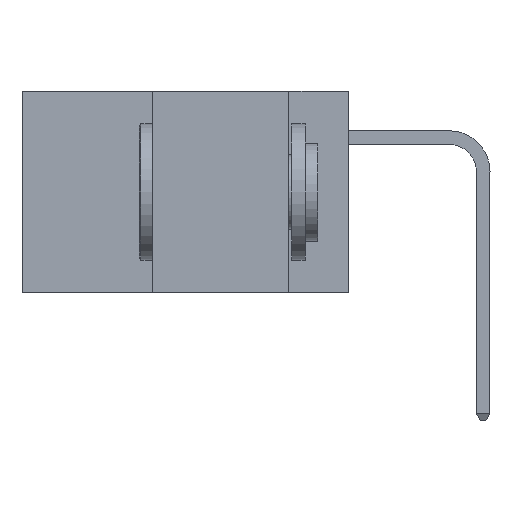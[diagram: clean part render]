
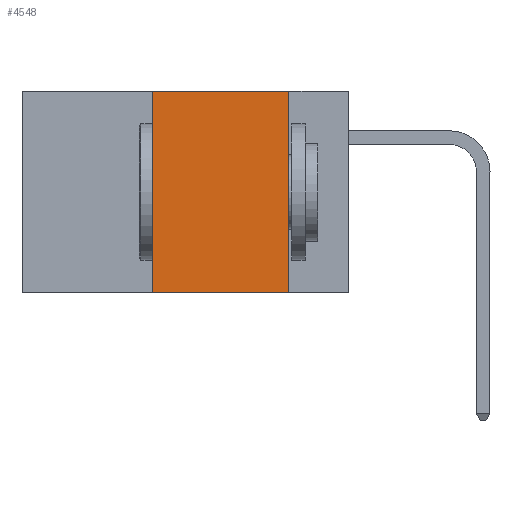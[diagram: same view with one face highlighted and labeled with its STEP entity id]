
A CAD part, left-side view. The second image highlights one B-rep face of the part: STEP entity #4548.
In plain terms, the highlighted planar face has unit normal (-1, 0, 0).
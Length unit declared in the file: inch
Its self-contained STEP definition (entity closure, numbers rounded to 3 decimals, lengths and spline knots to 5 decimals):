
#1615 = DIRECTION ( 'NONE',  ( 0., 0., -1. ) ) ;
#1675 = VECTOR ( 'NONE', #27861, 39.37008 ) ;
#3706 = LINE ( 'NONE', #6561, #33456 ) ;
#4021 = CARTESIAN_POINT ( 'NONE',  ( 0., 0.11, -0.37 ) ) ;
#4035 = CARTESIAN_POINT ( 'NONE',  ( 0., 0.11, 0. ) ) ;
#4548 = ADVANCED_FACE ( 'NONE', ( #15717 ), #34272, .F. ) ;
#5913 = ORIENTED_EDGE ( 'NONE', *, *, #23784, .T. ) ;
#6169 = VERTEX_POINT ( 'NONE', #30430 ) ;
#6561 = CARTESIAN_POINT ( 'NONE',  ( 0., 0.6, 0. ) ) ;
#9714 = VECTOR ( 'NONE', #33172, 39.37008 ) ;
#10504 = DIRECTION ( 'NONE',  ( 0., -1., 0. ) ) ;
#12415 = CARTESIAN_POINT ( 'NONE',  ( 0., 0.36, 0. ) ) ;
#12549 = DIRECTION ( 'NONE',  ( 0., -1., 0. ) ) ;
#13385 = EDGE_CURVE ( 'NONE', #16342, #17175, #18520, .T. ) ;
#13842 = CARTESIAN_POINT ( 'NONE',  ( 0., 0.36, 0. ) ) ;
#14933 = EDGE_LOOP ( 'NONE', ( #18956, #34711, #28713, #5913 ) ) ;
#15717 = FACE_OUTER_BOUND ( 'NONE', #14933, .T. ) ;
#15854 = VECTOR ( 'NONE', #10504, 39.37008 ) ;
#16342 = VERTEX_POINT ( 'NONE', #35878 ) ;
#16507 = CARTESIAN_POINT ( 'NONE',  ( 0., 0.6, 0. ) ) ;
#17175 = VERTEX_POINT ( 'NONE', #4021 ) ;
#18366 = EDGE_CURVE ( 'NONE', #6169, #35362, #31547, .T. ) ;
#18446 = AXIS2_PLACEMENT_3D ( 'NONE', #16507, #19540, #1615 ) ;
#18520 = LINE ( 'NONE', #4035, #1675 ) ;
#18956 = ORIENTED_EDGE ( 'NONE', *, *, #13385, .F. ) ;
#19540 = DIRECTION ( 'NONE',  ( 1., 0., 0. ) ) ;
#22362 = CARTESIAN_POINT ( 'NONE',  ( 0., 0.6, -0.37 ) ) ;
#23784 = EDGE_CURVE ( 'NONE', #6169, #17175, #30721, .T. ) ;
#27861 = DIRECTION ( 'NONE',  ( 0., 0., -1. ) ) ;
#28713 = ORIENTED_EDGE ( 'NONE', *, *, #18366, .F. ) ;
#30430 = CARTESIAN_POINT ( 'NONE',  ( 0., 0.36, -0.37 ) ) ;
#30721 = LINE ( 'NONE', #22362, #15854 ) ;
#31547 = LINE ( 'NONE', #12415, #9714 ) ;
#33172 = DIRECTION ( 'NONE',  ( 0., 0., 1. ) ) ;
#33456 = VECTOR ( 'NONE', #12549, 39.37008 ) ;
#34272 = PLANE ( 'NONE',  #18446 ) ;
#34711 = ORIENTED_EDGE ( 'NONE', *, *, #35092, .F. ) ;
#35092 = EDGE_CURVE ( 'NONE', #35362, #16342, #3706, .T. ) ;
#35362 = VERTEX_POINT ( 'NONE', #13842 ) ;
#35878 = CARTESIAN_POINT ( 'NONE',  ( 0., 0.11, 0. ) ) ;
